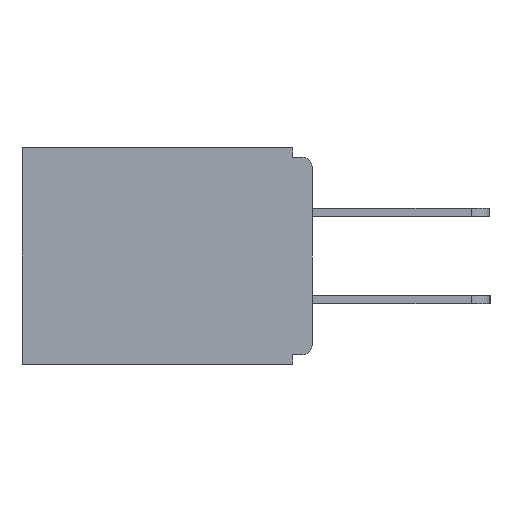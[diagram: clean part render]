
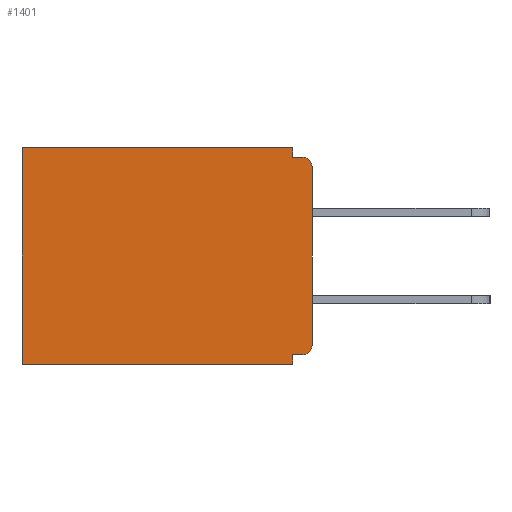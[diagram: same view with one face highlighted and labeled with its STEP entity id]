
A CAD part, left-side view. The second image highlights one B-rep face of the part: STEP entity #1401.
In plain terms, the highlighted planar face has unit normal (-1, 0, 0).
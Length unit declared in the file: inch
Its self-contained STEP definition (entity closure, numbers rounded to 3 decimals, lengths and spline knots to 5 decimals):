
#7 = CARTESIAN_POINT ( 'NONE',  ( 0.298, 0., 0. ) ) ;
#758 = FACE_OUTER_BOUND ( 'NONE', #3159, .T. ) ;
#960 = VERTEX_POINT ( 'NONE', #12797 ) ;
#1222 = DIRECTION ( 'NONE',  ( 0., 1., 0. ) ) ;
#1335 = AXIS2_PLACEMENT_3D ( 'NONE', #17746, #19167, #6755 ) ;
#1355 = VECTOR ( 'NONE', #14641, 39.37008 ) ;
#1401 = ADVANCED_FACE ( 'NONE', ( #758 ), #15589, .F. ) ;
#1413 = EDGE_CURVE ( 'NONE', #12800, #12813, #18582, .T. ) ;
#1470 = VERTEX_POINT ( 'NONE', #4533 ) ;
#2000 = LINE ( 'NONE', #10631, #19342 ) ;
#2086 = VERTEX_POINT ( 'NONE', #13299 ) ;
#2318 = LINE ( 'NONE', #8568, #1355 ) ;
#2446 = DIRECTION ( 'NONE',  ( 0., 0., -1. ) ) ;
#2893 = AXIS2_PLACEMENT_3D ( 'NONE', #5182, #11647, #8322 ) ;
#3132 = CARTESIAN_POINT ( 'NONE',  ( 0.298, 0., -0.343 ) ) ;
#3159 = EDGE_LOOP ( 'NONE', ( #5411, #3585, #4805, #14441, #4448, #18891, #3958, #4761, #16561, #3998 ) ) ;
#3547 = CARTESIAN_POINT ( 'NONE',  ( 0.298, 0., 0. ) ) ;
#3585 = ORIENTED_EDGE ( 'NONE', *, *, #7368, .F. ) ;
#3750 = CARTESIAN_POINT ( 'NONE',  ( 0.298, 0., 0. ) ) ;
#3958 = ORIENTED_EDGE ( 'NONE', *, *, #12632, .F. ) ;
#3998 = ORIENTED_EDGE ( 'NONE', *, *, #11932, .F. ) ;
#4448 = ORIENTED_EDGE ( 'NONE', *, *, #15736, .T. ) ;
#4454 = VECTOR ( 'NONE', #15848, 39.37008 ) ;
#4533 = CARTESIAN_POINT ( 'NONE',  ( 0.298, 0.015, -0.328 ) ) ;
#4761 = ORIENTED_EDGE ( 'NONE', *, *, #11807, .F. ) ;
#4805 = ORIENTED_EDGE ( 'NONE', *, *, #1413, .F. ) ;
#5182 = CARTESIAN_POINT ( 'NONE',  ( 0.298, 0.015, -0.313 ) ) ;
#5252 = CARTESIAN_POINT ( 'NONE',  ( 0.298, 0., -0.015 ) ) ;
#5411 = ORIENTED_EDGE ( 'NONE', *, *, #15879, .T. ) ;
#5983 = DIRECTION ( 'NONE',  ( 1., 0., 0. ) ) ;
#6407 = LINE ( 'NONE', #8733, #18360 ) ;
#6755 = DIRECTION ( 'NONE',  ( 0., 0., -1. ) ) ;
#7368 = EDGE_CURVE ( 'NONE', #12813, #11770, #7903, .T. ) ;
#7544 = DIRECTION ( 'NONE',  ( 0., 0., -1. ) ) ;
#7619 = DIRECTION ( 'NONE',  ( 0., 0., -1. ) ) ;
#7903 = LINE ( 'NONE', #5252, #16680 ) ;
#7969 = VERTEX_POINT ( 'NONE', #18206 ) ;
#8184 = CARTESIAN_POINT ( 'NONE',  ( 0.298, 0.031, -0.343 ) ) ;
#8322 = DIRECTION ( 'NONE',  ( 0., 0., -1. ) ) ;
#8568 = CARTESIAN_POINT ( 'NONE',  ( 0.298, 0.46, 0. ) ) ;
#8733 = CARTESIAN_POINT ( 'NONE',  ( 0.298, 0.031, -0.343 ) ) ;
#9293 = CARTESIAN_POINT ( 'NONE',  ( 0.298, 0.031, 0. ) ) ;
#9620 = LINE ( 'NONE', #3132, #4454 ) ;
#10370 = LINE ( 'NONE', #3547, #14986 ) ;
#10436 = VERTEX_POINT ( 'NONE', #8184 ) ;
#10631 = CARTESIAN_POINT ( 'NONE',  ( 0.298, 0., -0.328 ) ) ;
#11052 = VECTOR ( 'NONE', #7619, 39.37008 ) ;
#11624 = DIRECTION ( 'NONE',  ( 0., 1., 0. ) ) ;
#11647 = DIRECTION ( 'NONE',  ( -1., 0., 0. ) ) ;
#11770 = VERTEX_POINT ( 'NONE', #18435 ) ;
#11807 = EDGE_CURVE ( 'NONE', #1470, #15054, #2000, .T. ) ;
#11932 = EDGE_CURVE ( 'NONE', #2086, #7969, #10370, .T. ) ;
#12179 = VERTEX_POINT ( 'NONE', #15234 ) ;
#12632 = EDGE_CURVE ( 'NONE', #15054, #10436, #6407, .T. ) ;
#12797 = CARTESIAN_POINT ( 'NONE',  ( 0.298, 0.46, -0.343 ) ) ;
#12800 = VERTEX_POINT ( 'NONE', #9293 ) ;
#12813 = VERTEX_POINT ( 'NONE', #13712 ) ;
#12967 = DIRECTION ( 'NONE',  ( 0., -1., 0. ) ) ;
#13299 = CARTESIAN_POINT ( 'NONE',  ( 0.298, 0., -0.03 ) ) ;
#13409 = VECTOR ( 'NONE', #11624, 39.37008 ) ;
#13643 = DIRECTION ( 'NONE',  ( 0., 0., -1. ) ) ;
#13712 = CARTESIAN_POINT ( 'NONE',  ( 0.298, 0.031, -0.015 ) ) ;
#13833 = CARTESIAN_POINT ( 'NONE',  ( 0.298, 0.031, -0.343 ) ) ;
#14383 = EDGE_CURVE ( 'NONE', #1470, #7969, #18274, .T. ) ;
#14441 = ORIENTED_EDGE ( 'NONE', *, *, #14649, .T. ) ;
#14641 = DIRECTION ( 'NONE',  ( 0., 0., -1. ) ) ;
#14649 = EDGE_CURVE ( 'NONE', #12800, #12179, #17550, .T. ) ;
#14986 = VECTOR ( 'NONE', #2446, 39.37008 ) ;
#15054 = VERTEX_POINT ( 'NONE', #17391 ) ;
#15234 = CARTESIAN_POINT ( 'NONE',  ( 0.298, 0.46, 0. ) ) ;
#15589 = PLANE ( 'NONE',  #16129 ) ;
#15736 = EDGE_CURVE ( 'NONE', #12179, #960, #2318, .T. ) ;
#15848 = DIRECTION ( 'NONE',  ( 0., 1., 0. ) ) ;
#15879 = EDGE_CURVE ( 'NONE', #2086, #11770, #17011, .T. ) ;
#16129 = AXIS2_PLACEMENT_3D ( 'NONE', #7, #5983, #7544 ) ;
#16561 = ORIENTED_EDGE ( 'NONE', *, *, #14383, .T. ) ;
#16680 = VECTOR ( 'NONE', #12967, 39.37008 ) ;
#17011 = CIRCLE ( 'NONE', #1335, 0.015 ) ;
#17391 = CARTESIAN_POINT ( 'NONE',  ( 0.298, 0.031, -0.328 ) ) ;
#17550 = LINE ( 'NONE', #3750, #13409 ) ;
#17746 = CARTESIAN_POINT ( 'NONE',  ( 0.298, 0.015, -0.03 ) ) ;
#17760 = EDGE_CURVE ( 'NONE', #10436, #960, #9620, .T. ) ;
#18206 = CARTESIAN_POINT ( 'NONE',  ( 0.298, 0., -0.313 ) ) ;
#18274 = CIRCLE ( 'NONE', #2893, 0.015 ) ;
#18360 = VECTOR ( 'NONE', #13643, 39.37008 ) ;
#18435 = CARTESIAN_POINT ( 'NONE',  ( 0.298, 0.015, -0.015 ) ) ;
#18582 = LINE ( 'NONE', #13833, #11052 ) ;
#18891 = ORIENTED_EDGE ( 'NONE', *, *, #17760, .F. ) ;
#19167 = DIRECTION ( 'NONE',  ( -1., 0., 0. ) ) ;
#19342 = VECTOR ( 'NONE', #1222, 39.37008 ) ;
